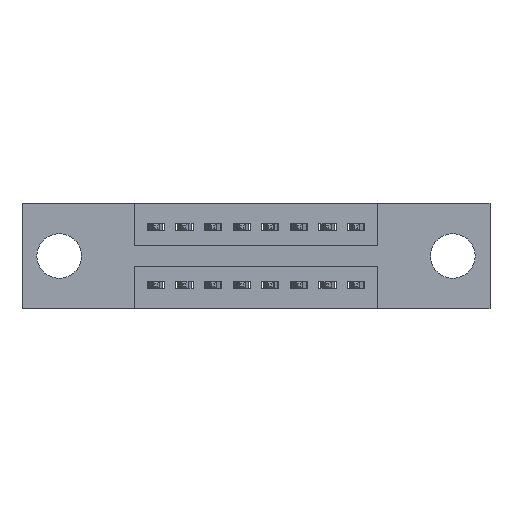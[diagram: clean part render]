
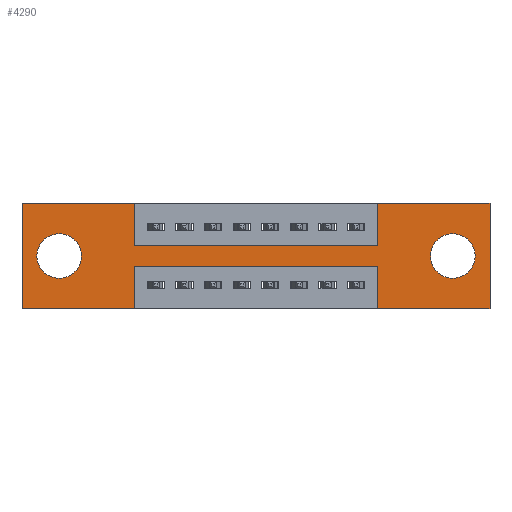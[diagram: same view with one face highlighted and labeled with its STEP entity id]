
A CAD part, front view. The second image highlights one B-rep face of the part: STEP entity #4290.
In plain terms, the highlighted planar face has unit normal (0, -1, 0).
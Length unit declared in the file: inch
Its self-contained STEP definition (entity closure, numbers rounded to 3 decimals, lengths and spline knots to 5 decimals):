
#12 = ORIENTED_EDGE ( 'NONE', *, *, #6829, .F. ) ;
#58 = FACE_BOUND ( 'NONE', #67, .T. ) ;
#67 = EDGE_LOOP ( 'NONE', ( #9849, #9935 ) ) ;
#114 = ORIENTED_EDGE ( 'NONE', *, *, #8990, .F. ) ;
#129 = VERTEX_POINT ( 'NONE', #1044 ) ;
#215 = EDGE_CURVE ( 'NONE', #2121, #10642, #6250, .T. ) ;
#218 = EDGE_LOOP ( 'NONE', ( #9947, #9968 ) ) ;
#314 = DIRECTION ( 'NONE',  ( -1., 0., 0. ) ) ;
#605 = VERTEX_POINT ( 'NONE', #10824 ) ;
#627 = CIRCLE ( 'NONE', #10040, 0.078 ) ;
#646 = LINE ( 'NONE', #1836, #7605 ) ;
#672 = LINE ( 'NONE', #7415, #9673 ) ;
#696 = VERTEX_POINT ( 'NONE', #4314 ) ;
#720 = ORIENTED_EDGE ( 'NONE', *, *, #1533, .F. ) ;
#728 = ORIENTED_EDGE ( 'NONE', *, *, #6802, .F. ) ;
#775 = AXIS2_PLACEMENT_3D ( 'NONE', #4322, #10209, #5266 ) ;
#786 = EDGE_CURVE ( 'NONE', #129, #2317, #3826, .T. ) ;
#787 = CARTESIAN_POINT ( 'NONE',  ( 0.13, 0., -0.107 ) ) ;
#1044 = CARTESIAN_POINT ( 'NONE',  ( 1.2425, 0., -0.22 ) ) ;
#1121 = EDGE_CURVE ( 'NONE', #5018, #2121, #10156, .T. ) ;
#1169 = VERTEX_POINT ( 'NONE', #6337 ) ;
#1281 = ORIENTED_EDGE ( 'NONE', *, *, #8045, .F. ) ;
#1333 = EDGE_CURVE ( 'NONE', #3766, #129, #4358, .T. ) ;
#1352 = ORIENTED_EDGE ( 'NONE', *, *, #6552, .F. ) ;
#1511 = CARTESIAN_POINT ( 'NONE',  ( 0.13, 0., -0.263 ) ) ;
#1533 = EDGE_CURVE ( 'NONE', #8130, #605, #9036, .T. ) ;
#1545 = DIRECTION ( 'NONE',  ( 0., 0., -1. ) ) ;
#1560 = VECTOR ( 'NONE', #3167, 39.37008 ) ;
#1626 = PLANE ( 'NONE',  #9250 ) ;
#1636 = CARTESIAN_POINT ( 'NONE',  ( 0., 0., -0.37 ) ) ;
#1781 = CARTESIAN_POINT ( 'NONE',  ( 1.505, 0., -0.185 ) ) ;
#1787 = DIRECTION ( 'NONE',  ( 0., -1., 0. ) ) ;
#1829 = DIRECTION ( 'NONE',  ( -1., 0., 0. ) ) ;
#1836 = CARTESIAN_POINT ( 'NONE',  ( 0.3925, 0., -0.37 ) ) ;
#1882 = CARTESIAN_POINT ( 'NONE',  ( 0.3925, 0., 0. ) ) ;
#1907 = DIRECTION ( 'NONE',  ( 0., 0., -1. ) ) ;
#1922 = CARTESIAN_POINT ( 'NONE',  ( 1.635, 0., 0. ) ) ;
#2025 = CIRCLE ( 'NONE', #9831, 0.078 ) ;
#2049 = FACE_OUTER_BOUND ( 'NONE', #5003, .T. ) ;
#2121 = VERTEX_POINT ( 'NONE', #7771 ) ;
#2124 = DIRECTION ( 'NONE',  ( 1., 0., 0. ) ) ;
#2157 = DIRECTION ( 'NONE',  ( 0., 0., 1. ) ) ;
#2210 = VECTOR ( 'NONE', #1907, 39.37008 ) ;
#2254 = VERTEX_POINT ( 'NONE', #1511 ) ;
#2278 = CARTESIAN_POINT ( 'NONE',  ( 1.505, 0., -0.185 ) ) ;
#2317 = VERTEX_POINT ( 'NONE', #8664 ) ;
#2615 = EDGE_CURVE ( 'NONE', #2317, #8506, #646, .T. ) ;
#2624 = DIRECTION ( 'NONE',  ( 0., 1., 0. ) ) ;
#2634 = DIRECTION ( 'NONE',  ( 1., 0., 0. ) ) ;
#2637 = DIRECTION ( 'NONE',  ( 0., 0., -1. ) ) ;
#2686 = CARTESIAN_POINT ( 'NONE',  ( 1.505, 0., -0.263 ) ) ;
#2741 = CARTESIAN_POINT ( 'NONE',  ( 1.635, 0., -0.37 ) ) ;
#2777 = LINE ( 'NONE', #7115, #4826 ) ;
#2804 = VERTEX_POINT ( 'NONE', #787 ) ;
#3126 = DIRECTION ( 'NONE',  ( 0., 0., -1. ) ) ;
#3167 = DIRECTION ( 'NONE',  ( -1., 0., 0. ) ) ;
#3289 = DIRECTION ( 'NONE',  ( 0., 0., 1. ) ) ;
#3766 = VERTEX_POINT ( 'NONE', #6659 ) ;
#3826 = LINE ( 'NONE', #6079, #1560 ) ;
#3836 = VECTOR ( 'NONE', #8768, 39.37008 ) ;
#3927 = DIRECTION ( 'NONE',  ( 0., 0., 1. ) ) ;
#4031 = LINE ( 'NONE', #10411, #8652 ) ;
#4067 = LINE ( 'NONE', #8272, #4347 ) ;
#4290 = ADVANCED_FACE ( 'NONE', ( #58, #6467, #2049 ), #1626, .T. ) ;
#4314 = CARTESIAN_POINT ( 'NONE',  ( 1.505, 0., -0.107 ) ) ;
#4322 = CARTESIAN_POINT ( 'NONE',  ( 0.13, 0., -0.185 ) ) ;
#4347 = VECTOR ( 'NONE', #3927, 39.37008 ) ;
#4358 = LINE ( 'NONE', #7798, #10270 ) ;
#4389 = AXIS2_PLACEMENT_3D ( 'NONE', #7906, #2624, #8657 ) ;
#4826 = VECTOR ( 'NONE', #1829, 39.37008 ) ;
#5003 = EDGE_LOOP ( 'NONE', ( #10027, #10050, #10288, #10335, #10500, #10536, #12, #114, #720, #728, #1281, #1352 ) ) ;
#5018 = VERTEX_POINT ( 'NONE', #10518 ) ;
#5266 = DIRECTION ( 'NONE',  ( 0., 0., 1. ) ) ;
#5787 = VECTOR ( 'NONE', #2634, 39.37008 ) ;
#6079 = CARTESIAN_POINT ( 'NONE',  ( 0.3925, 0., -0.22 ) ) ;
#6226 = CARTESIAN_POINT ( 'NONE',  ( 0., 0., 0. ) ) ;
#6250 = LINE ( 'NONE', #1922, #3836 ) ;
#6337 = CARTESIAN_POINT ( 'NONE',  ( 0., 0., 0. ) ) ;
#6467 = FACE_BOUND ( 'NONE', #218, .T. ) ;
#6552 = EDGE_CURVE ( 'NONE', #8506, #9384, #2777, .T. ) ;
#6596 = CIRCLE ( 'NONE', #775, 0.078 ) ;
#6659 = CARTESIAN_POINT ( 'NONE',  ( 1.2425, 0., -0.37 ) ) ;
#6729 = LINE ( 'NONE', #10682, #8663 ) ;
#6776 = LINE ( 'NONE', #8252, #7373 ) ;
#6802 = EDGE_CURVE ( 'NONE', #1169, #8130, #672, .T. ) ;
#6829 = EDGE_CURVE ( 'NONE', #8131, #5018, #6776, .T. ) ;
#7115 = CARTESIAN_POINT ( 'NONE',  ( 0., 0., -0.37 ) ) ;
#7154 = CARTESIAN_POINT ( 'NONE',  ( 0., 0., -0.37 ) ) ;
#7327 = CIRCLE ( 'NONE', #4389, 0.078 ) ;
#7373 = VECTOR ( 'NONE', #2157, 39.37008 ) ;
#7392 = DIRECTION ( 'NONE',  ( 0., 0., -1. ) ) ;
#7415 = CARTESIAN_POINT ( 'NONE',  ( 0., 0., 0. ) ) ;
#7605 = VECTOR ( 'NONE', #7392, 39.37008 ) ;
#7771 = CARTESIAN_POINT ( 'NONE',  ( 1.635, 0., 0. ) ) ;
#7798 = CARTESIAN_POINT ( 'NONE',  ( 1.2425, 0., -0.37 ) ) ;
#7906 = CARTESIAN_POINT ( 'NONE',  ( 0.13, 0., -0.185 ) ) ;
#7916 = DIRECTION ( 'NONE',  ( 0., 1., 0. ) ) ;
#8045 = EDGE_CURVE ( 'NONE', #9384, #1169, #4067, .T. ) ;
#8130 = VERTEX_POINT ( 'NONE', #9121 ) ;
#8131 = VERTEX_POINT ( 'NONE', #9918 ) ;
#8252 = CARTESIAN_POINT ( 'NONE',  ( 1.2425, 0., 0. ) ) ;
#8272 = CARTESIAN_POINT ( 'NONE',  ( 0., 0., 0. ) ) ;
#8358 = DIRECTION ( 'NONE',  ( 0., 1., 0. ) ) ;
#8434 = EDGE_CURVE ( 'NONE', #2804, #2254, #7327, .T. ) ;
#8506 = VERTEX_POINT ( 'NONE', #10255 ) ;
#8652 = VECTOR ( 'NONE', #314, 39.37008 ) ;
#8657 = DIRECTION ( 'NONE',  ( 0., 0., 1. ) ) ;
#8663 = VECTOR ( 'NONE', #9144, 39.37008 ) ;
#8664 = CARTESIAN_POINT ( 'NONE',  ( 0.3925, 0., -0.22 ) ) ;
#8768 = DIRECTION ( 'NONE',  ( 0., 0., -1. ) ) ;
#8936 = EDGE_CURVE ( 'NONE', #696, #9365, #627, .T. ) ;
#8990 = EDGE_CURVE ( 'NONE', #605, #8131, #6729, .T. ) ;
#9036 = LINE ( 'NONE', #1882, #2210 ) ;
#9121 = CARTESIAN_POINT ( 'NONE',  ( 0.3925, 0., 0. ) ) ;
#9144 = DIRECTION ( 'NONE',  ( 1., 0., 0. ) ) ;
#9250 = AXIS2_PLACEMENT_3D ( 'NONE', #1636, #1787, #1545 ) ;
#9283 = EDGE_CURVE ( 'NONE', #2254, #2804, #6596, .T. ) ;
#9365 = VERTEX_POINT ( 'NONE', #2686 ) ;
#9384 = VERTEX_POINT ( 'NONE', #7154 ) ;
#9535 = EDGE_CURVE ( 'NONE', #10642, #3766, #4031, .T. ) ;
#9673 = VECTOR ( 'NONE', #2124, 39.37008 ) ;
#9831 = AXIS2_PLACEMENT_3D ( 'NONE', #1781, #7916, #2637 ) ;
#9849 = ORIENTED_EDGE ( 'NONE', *, *, #8936, .T. ) ;
#9918 = CARTESIAN_POINT ( 'NONE',  ( 1.2425, 0., -0.15 ) ) ;
#9935 = ORIENTED_EDGE ( 'NONE', *, *, #10521, .T. ) ;
#9947 = ORIENTED_EDGE ( 'NONE', *, *, #8434, .T. ) ;
#9968 = ORIENTED_EDGE ( 'NONE', *, *, #9283, .T. ) ;
#10027 = ORIENTED_EDGE ( 'NONE', *, *, #2615, .F. ) ;
#10040 = AXIS2_PLACEMENT_3D ( 'NONE', #2278, #8358, #3126 ) ;
#10050 = ORIENTED_EDGE ( 'NONE', *, *, #786, .F. ) ;
#10156 = LINE ( 'NONE', #6226, #5787 ) ;
#10209 = DIRECTION ( 'NONE',  ( 0., 1., 0. ) ) ;
#10255 = CARTESIAN_POINT ( 'NONE',  ( 0.3925, 0., -0.37 ) ) ;
#10270 = VECTOR ( 'NONE', #3289, 39.37008 ) ;
#10288 = ORIENTED_EDGE ( 'NONE', *, *, #1333, .F. ) ;
#10335 = ORIENTED_EDGE ( 'NONE', *, *, #9535, .F. ) ;
#10411 = CARTESIAN_POINT ( 'NONE',  ( 0., 0., -0.37 ) ) ;
#10500 = ORIENTED_EDGE ( 'NONE', *, *, #215, .F. ) ;
#10518 = CARTESIAN_POINT ( 'NONE',  ( 1.2425, 0., 0. ) ) ;
#10521 = EDGE_CURVE ( 'NONE', #9365, #696, #2025, .T. ) ;
#10536 = ORIENTED_EDGE ( 'NONE', *, *, #1121, .F. ) ;
#10642 = VERTEX_POINT ( 'NONE', #2741 ) ;
#10682 = CARTESIAN_POINT ( 'NONE',  ( 0.3925, 0., -0.15 ) ) ;
#10824 = CARTESIAN_POINT ( 'NONE',  ( 0.3925, 0., -0.15 ) ) ;
